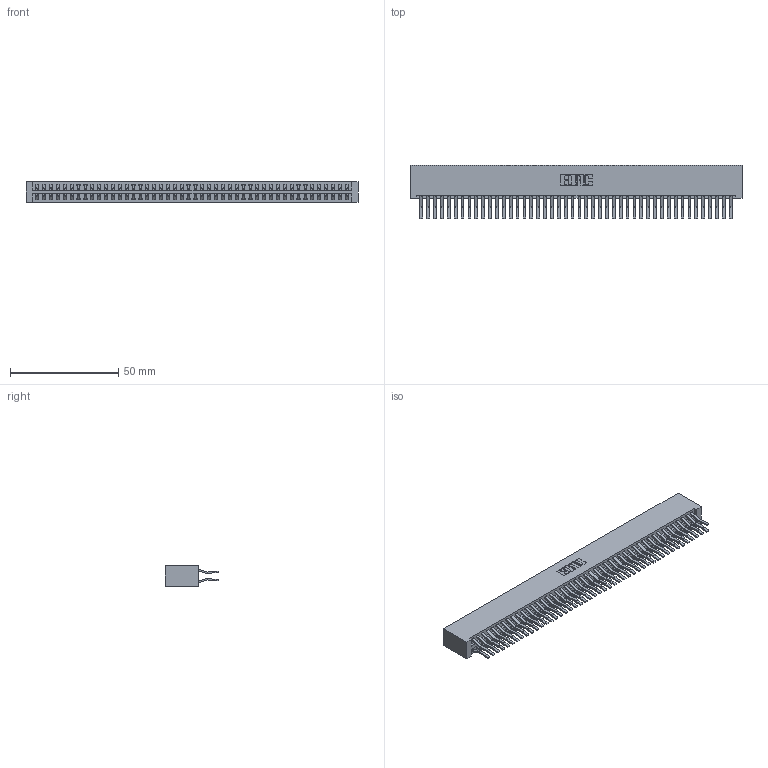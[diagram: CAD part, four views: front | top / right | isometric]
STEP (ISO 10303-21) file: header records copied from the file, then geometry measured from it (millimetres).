
FILE_DESCRIPTION (( 'STEP AP203' ), '1' );
FILE_NAME ('346-092-560-201.STEP', '2022-05-26T08:43:19', ( '' ), ( '' ), 'SwSTEP 2.0', 'SolidWorks 2020', '' );
FILE_SCHEMA (( 'CONFIG_CONTROL_DESIGN' ));
Length unit declared in the file: inch
Products named in the file (3): 346-092-560-201; 345-292-001_560 Tail; 346 Part_No Mounting Lugs
Assembly tree (93 placements, depth 2):
  346-092-560-201
    346 Part_No Mounting Lugs
    345-292-001_560 Tail  x92
Bounding box: 153.29 x 24.78 x 9.4 mm (x, y, z)
Volume: 16155 mm3; surface area: 24041 mm2
Topology: 93 solids, 93 shells, 5082 faces, 15117 edges, 9954 vertices
Faces by surface type: plane 3292, cylinder 1790
Entity records: 29293 total; most frequent: CARTESIAN_POINT 4820, ORIENTED_EDGE 4754, DIRECTION 4297, EDGE_CURVE 2377, LINE 2065, VECTOR 2065, VERTEX_POINT 1582, AXIS2_PLACEMENT_3D 1116
